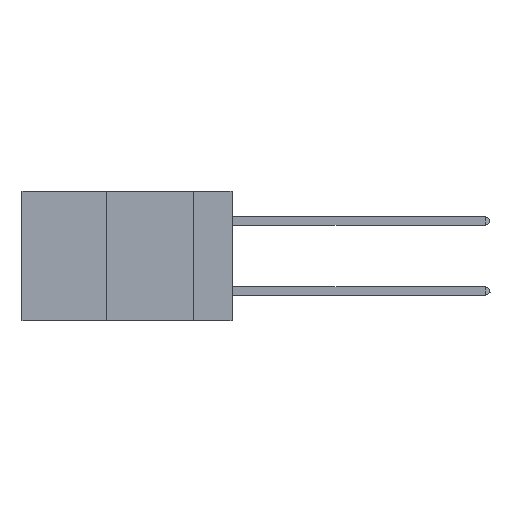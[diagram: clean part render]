
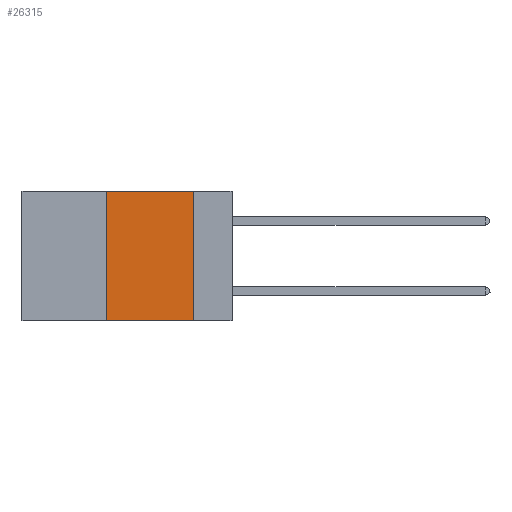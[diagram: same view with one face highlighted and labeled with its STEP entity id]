
A CAD part, left-side view. The second image highlights one B-rep face of the part: STEP entity #26315.
In plain terms, the highlighted planar face has unit normal (-1, 0, 0).
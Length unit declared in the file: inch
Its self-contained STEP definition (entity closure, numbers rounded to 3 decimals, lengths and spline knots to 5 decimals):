
#562 = CARTESIAN_POINT ( 'NONE',  ( 0., 0.6, 0. ) ) ;
#1058 = LINE ( 'NONE', #3083, #14100 ) ;
#1755 = DIRECTION ( 'NONE',  ( 0., -1., 0. ) ) ;
#2739 = CARTESIAN_POINT ( 'NONE',  ( 0., 0.11, -0.37 ) ) ;
#3083 = CARTESIAN_POINT ( 'NONE',  ( 0., 0.36, 0. ) ) ;
#4063 = LINE ( 'NONE', #6485, #20182 ) ;
#4984 = VERTEX_POINT ( 'NONE', #19155 ) ;
#6485 = CARTESIAN_POINT ( 'NONE',  ( 0., 0.11, 0. ) ) ;
#9012 = CARTESIAN_POINT ( 'NONE',  ( 0., 0.6, 0. ) ) ;
#10215 = VERTEX_POINT ( 'NONE', #2739 ) ;
#10524 = LINE ( 'NONE', #562, #14998 ) ;
#11433 = LINE ( 'NONE', #21234, #25829 ) ;
#13693 = CARTESIAN_POINT ( 'NONE',  ( 0., 0.36, -0.37 ) ) ;
#14100 = VECTOR ( 'NONE', #22839, 39.37008 ) ;
#14998 = VECTOR ( 'NONE', #20195, 39.37008 ) ;
#18065 = DIRECTION ( 'NONE',  ( 0., 0., -1. ) ) ;
#18896 = ORIENTED_EDGE ( 'NONE', *, *, #20458, .T. ) ;
#19155 = CARTESIAN_POINT ( 'NONE',  ( 0., 0.36, 0. ) ) ;
#20177 = VERTEX_POINT ( 'NONE', #13693 ) ;
#20182 = VECTOR ( 'NONE', #23825, 39.37008 ) ;
#20195 = DIRECTION ( 'NONE',  ( 0., -1., 0. ) ) ;
#20458 = EDGE_CURVE ( 'NONE', #20177, #10215, #11433, .T. ) ;
#20827 = CARTESIAN_POINT ( 'NONE',  ( 0., 0.11, 0. ) ) ;
#21234 = CARTESIAN_POINT ( 'NONE',  ( 0., 0.6, -0.37 ) ) ;
#22011 = VERTEX_POINT ( 'NONE', #20827 ) ;
#22265 = DIRECTION ( 'NONE',  ( 1., 0., 0. ) ) ;
#22348 = ORIENTED_EDGE ( 'NONE', *, *, #27599, .F. ) ;
#22839 = DIRECTION ( 'NONE',  ( 0., 0., 1. ) ) ;
#23099 = EDGE_CURVE ( 'NONE', #4984, #22011, #10524, .T. ) ;
#23825 = DIRECTION ( 'NONE',  ( 0., 0., -1. ) ) ;
#24732 = PLANE ( 'NONE',  #26964 ) ;
#25803 = EDGE_LOOP ( 'NONE', ( #22348, #26862, #26042, #18896 ) ) ;
#25829 = VECTOR ( 'NONE', #1755, 39.37008 ) ;
#26042 = ORIENTED_EDGE ( 'NONE', *, *, #26390, .F. ) ;
#26315 = ADVANCED_FACE ( 'NONE', ( #27103 ), #24732, .F. ) ;
#26390 = EDGE_CURVE ( 'NONE', #20177, #4984, #1058, .T. ) ;
#26862 = ORIENTED_EDGE ( 'NONE', *, *, #23099, .F. ) ;
#26964 = AXIS2_PLACEMENT_3D ( 'NONE', #9012, #22265, #18065 ) ;
#27103 = FACE_OUTER_BOUND ( 'NONE', #25803, .T. ) ;
#27599 = EDGE_CURVE ( 'NONE', #22011, #10215, #4063, .T. ) ;
